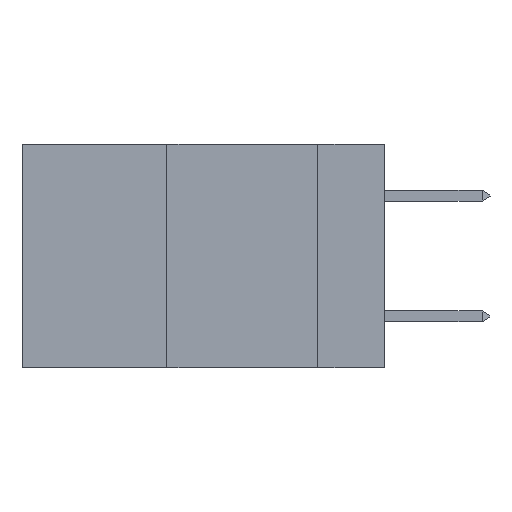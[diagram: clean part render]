
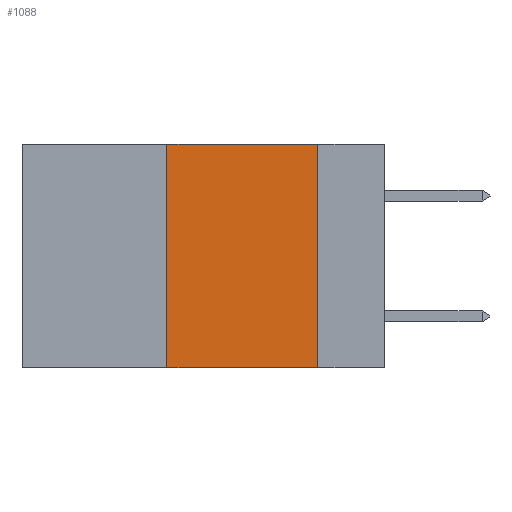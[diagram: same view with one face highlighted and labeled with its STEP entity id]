
A CAD part, left-side view. The second image highlights one B-rep face of the part: STEP entity #1088.
In plain terms, the highlighted planar face has unit normal (-1, 0, 0).
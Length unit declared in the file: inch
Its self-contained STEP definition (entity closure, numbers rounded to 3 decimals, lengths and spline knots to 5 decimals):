
#206 = AXIS2_PLACEMENT_3D ( 'NONE', #3418, #7201, #7286 ) ;
#297 = CARTESIAN_POINT ( 'NONE',  ( 0., 0.11, -0.37 ) ) ;
#452 = PLANE ( 'NONE',  #206 ) ;
#587 = DIRECTION ( 'NONE',  ( 0., 0., -1. ) ) ;
#1088 = ADVANCED_FACE ( 'NONE', ( #7099 ), #452, .F. ) ;
#1346 = CARTESIAN_POINT ( 'NONE',  ( 0., 0.11, 0. ) ) ;
#1466 = CARTESIAN_POINT ( 'NONE',  ( 0., 0.36, -0.37 ) ) ;
#1887 = VECTOR ( 'NONE', #7801, 39.37008 ) ;
#2136 = VERTEX_POINT ( 'NONE', #1346 ) ;
#2638 = CARTESIAN_POINT ( 'NONE',  ( 0., 0.6, -0.37 ) ) ;
#2657 = ORIENTED_EDGE ( 'NONE', *, *, #8386, .F. ) ;
#3135 = LINE ( 'NONE', #8916, #7608 ) ;
#3195 = CARTESIAN_POINT ( 'NONE',  ( 0., 0.6, 0. ) ) ;
#3412 = LINE ( 'NONE', #2638, #7006 ) ;
#3418 = CARTESIAN_POINT ( 'NONE',  ( 0., 0.6, 0. ) ) ;
#3537 = VECTOR ( 'NONE', #587, 39.37008 ) ;
#4352 = EDGE_CURVE ( 'NONE', #2136, #5323, #8698, .T. ) ;
#4398 = DIRECTION ( 'NONE',  ( 0., 0., 1. ) ) ;
#5323 = VERTEX_POINT ( 'NONE', #297 ) ;
#5671 = VERTEX_POINT ( 'NONE', #9444 ) ;
#5678 = CARTESIAN_POINT ( 'NONE',  ( 0., 0.11, 0. ) ) ;
#6016 = ORIENTED_EDGE ( 'NONE', *, *, #4352, .F. ) ;
#6378 = VERTEX_POINT ( 'NONE', #1466 ) ;
#7006 = VECTOR ( 'NONE', #7868, 39.37008 ) ;
#7099 = FACE_OUTER_BOUND ( 'NONE', #7217, .T. ) ;
#7201 = DIRECTION ( 'NONE',  ( 1., 0., 0. ) ) ;
#7217 = EDGE_LOOP ( 'NONE', ( #6016, #2657, #9075, #9082 ) ) ;
#7286 = DIRECTION ( 'NONE',  ( 0., 0., -1. ) ) ;
#7608 = VECTOR ( 'NONE', #4398, 39.37008 ) ;
#7691 = LINE ( 'NONE', #3195, #1887 ) ;
#7801 = DIRECTION ( 'NONE',  ( 0., -1., 0. ) ) ;
#7868 = DIRECTION ( 'NONE',  ( 0., -1., 0. ) ) ;
#8386 = EDGE_CURVE ( 'NONE', #5671, #2136, #7691, .T. ) ;
#8698 = LINE ( 'NONE', #5678, #3537 ) ;
#8735 = EDGE_CURVE ( 'NONE', #6378, #5671, #3135, .T. ) ;
#8916 = CARTESIAN_POINT ( 'NONE',  ( 0., 0.36, 0. ) ) ;
#9075 = ORIENTED_EDGE ( 'NONE', *, *, #8735, .F. ) ;
#9082 = ORIENTED_EDGE ( 'NONE', *, *, #9431, .T. ) ;
#9431 = EDGE_CURVE ( 'NONE', #6378, #5323, #3412, .T. ) ;
#9444 = CARTESIAN_POINT ( 'NONE',  ( 0., 0.36, 0. ) ) ;
